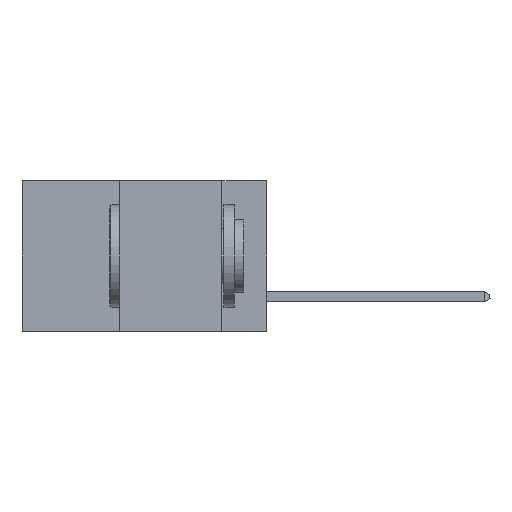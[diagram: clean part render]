
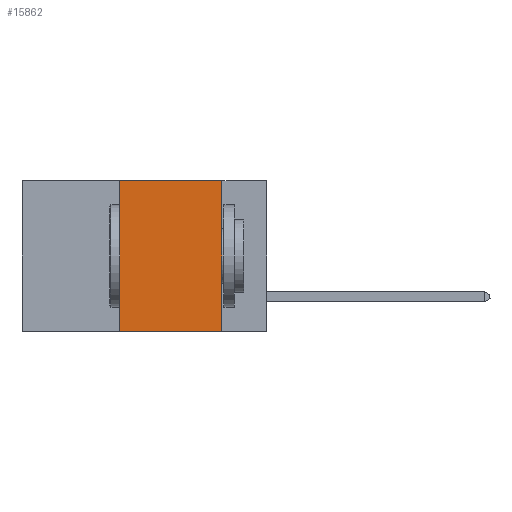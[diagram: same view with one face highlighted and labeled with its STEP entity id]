
A CAD part, left-side view. The second image highlights one B-rep face of the part: STEP entity #15862.
In plain terms, the highlighted planar face has unit normal (-1, 0, 0).
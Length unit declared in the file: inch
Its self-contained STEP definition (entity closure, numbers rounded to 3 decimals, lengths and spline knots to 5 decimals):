
#21 = CARTESIAN_POINT ( 'NONE',  ( 0., 0.11, 0. ) ) ;
#539 = EDGE_CURVE ( 'NONE', #6673, #5004, #11190, .T. ) ;
#1405 = EDGE_CURVE ( 'NONE', #6673, #9666, #10404, .T. ) ;
#1733 = DIRECTION ( 'NONE',  ( 0., 0., -1. ) ) ;
#2282 = EDGE_CURVE ( 'NONE', #11222, #5004, #3301, .T. ) ;
#2486 = EDGE_LOOP ( 'NONE', ( #8419, #15826, #5701, #11320 ) ) ;
#2753 = DIRECTION ( 'NONE',  ( 0., -1., 0. ) ) ;
#3301 = LINE ( 'NONE', #21, #6717 ) ;
#3319 = CARTESIAN_POINT ( 'NONE',  ( 0., 0.11, 0. ) ) ;
#3795 = LINE ( 'NONE', #13736, #6779 ) ;
#5004 = VERTEX_POINT ( 'NONE', #8552 ) ;
#5670 = CARTESIAN_POINT ( 'NONE',  ( 0., 0.6, 0. ) ) ;
#5701 = ORIENTED_EDGE ( 'NONE', *, *, #1405, .F. ) ;
#6274 = DIRECTION ( 'NONE',  ( 0., 0., 1. ) ) ;
#6673 = VERTEX_POINT ( 'NONE', #9471 ) ;
#6717 = VECTOR ( 'NONE', #1733, 39.37008 ) ;
#6779 = VECTOR ( 'NONE', #14981, 39.37008 ) ;
#6948 = DIRECTION ( 'NONE',  ( 1., 0., 0. ) ) ;
#7150 = VECTOR ( 'NONE', #6274, 39.37008 ) ;
#8110 = CARTESIAN_POINT ( 'NONE',  ( 0., 0.36, 0. ) ) ;
#8419 = ORIENTED_EDGE ( 'NONE', *, *, #2282, .F. ) ;
#8552 = CARTESIAN_POINT ( 'NONE',  ( 0., 0.11, -0.37 ) ) ;
#9471 = CARTESIAN_POINT ( 'NONE',  ( 0., 0.36, -0.37 ) ) ;
#9666 = VERTEX_POINT ( 'NONE', #13733 ) ;
#10404 = LINE ( 'NONE', #8110, #7150 ) ;
#11190 = LINE ( 'NONE', #12140, #14077 ) ;
#11222 = VERTEX_POINT ( 'NONE', #3319 ) ;
#11320 = ORIENTED_EDGE ( 'NONE', *, *, #539, .T. ) ;
#11446 = EDGE_CURVE ( 'NONE', #9666, #11222, #3795, .T. ) ;
#12140 = CARTESIAN_POINT ( 'NONE',  ( 0., 0.6, -0.37 ) ) ;
#13576 = AXIS2_PLACEMENT_3D ( 'NONE', #5670, #6948, #15563 ) ;
#13733 = CARTESIAN_POINT ( 'NONE',  ( 0., 0.36, 0. ) ) ;
#13736 = CARTESIAN_POINT ( 'NONE',  ( 0., 0.6, 0. ) ) ;
#14077 = VECTOR ( 'NONE', #2753, 39.37008 ) ;
#14248 = PLANE ( 'NONE',  #13576 ) ;
#14981 = DIRECTION ( 'NONE',  ( 0., -1., 0. ) ) ;
#15302 = FACE_OUTER_BOUND ( 'NONE', #2486, .T. ) ;
#15563 = DIRECTION ( 'NONE',  ( 0., 0., -1. ) ) ;
#15826 = ORIENTED_EDGE ( 'NONE', *, *, #11446, .F. ) ;
#15862 = ADVANCED_FACE ( 'NONE', ( #15302 ), #14248, .F. ) ;
